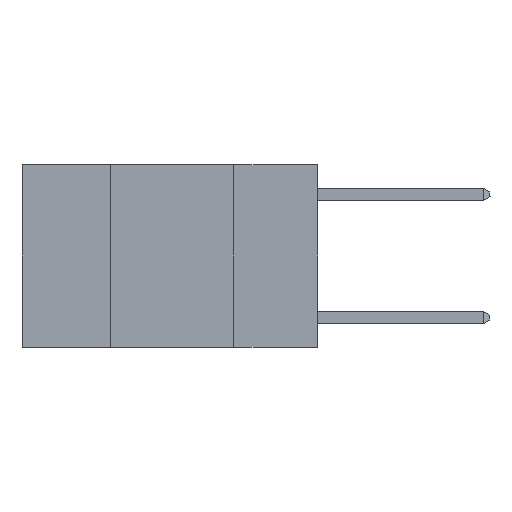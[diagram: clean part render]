
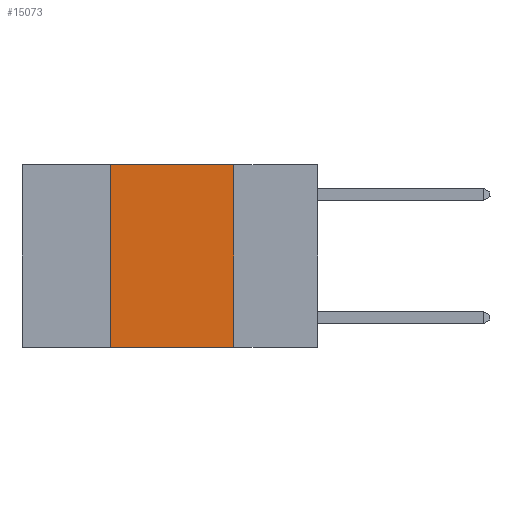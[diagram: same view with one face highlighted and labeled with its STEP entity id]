
A CAD part, left-side view. The second image highlights one B-rep face of the part: STEP entity #15073.
In plain terms, the highlighted planar face has unit normal (-1, 0, 0).
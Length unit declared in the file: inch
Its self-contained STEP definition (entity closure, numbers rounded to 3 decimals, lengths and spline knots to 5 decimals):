
#300 = VECTOR ( 'NONE', #2302, 39.37008 ) ;
#547 = EDGE_CURVE ( 'NONE', #1312, #9649, #878, .T. ) ;
#878 = LINE ( 'NONE', #14777, #6527 ) ;
#1312 = VERTEX_POINT ( 'NONE', #2654 ) ;
#1399 = EDGE_CURVE ( 'NONE', #7088, #1312, #10893, .T. ) ;
#1796 = CARTESIAN_POINT ( 'NONE',  ( 0., 0.6, -0.37 ) ) ;
#2073 = ORIENTED_EDGE ( 'NONE', *, *, #9136, .T. ) ;
#2124 = ORIENTED_EDGE ( 'NONE', *, *, #1399, .F. ) ;
#2302 = DIRECTION ( 'NONE',  ( 0., -1., 0. ) ) ;
#2654 = CARTESIAN_POINT ( 'NONE',  ( 0., 0.17, 0. ) ) ;
#2796 = EDGE_CURVE ( 'NONE', #14034, #7088, #12800, .T. ) ;
#3447 = DIRECTION ( 'NONE',  ( 0., 0., 1. ) ) ;
#3804 = AXIS2_PLACEMENT_3D ( 'NONE', #9010, #4332, #12640 ) ;
#4332 = DIRECTION ( 'NONE',  ( 1., 0., 0. ) ) ;
#4443 = EDGE_LOOP ( 'NONE', ( #9001, #2124, #13896, #2073 ) ) ;
#5183 = DIRECTION ( 'NONE',  ( 0., 0., -1. ) ) ;
#6338 = CARTESIAN_POINT ( 'NONE',  ( 0., 0.42, 0. ) ) ;
#6527 = VECTOR ( 'NONE', #5183, 39.37008 ) ;
#7088 = VERTEX_POINT ( 'NONE', #8324 ) ;
#7372 = VECTOR ( 'NONE', #12510, 39.37008 ) ;
#7829 = PLANE ( 'NONE',  #3804 ) ;
#8324 = CARTESIAN_POINT ( 'NONE',  ( 0., 0.42, 0. ) ) ;
#9001 = ORIENTED_EDGE ( 'NONE', *, *, #547, .F. ) ;
#9010 = CARTESIAN_POINT ( 'NONE',  ( 0., 0.6, 0. ) ) ;
#9136 = EDGE_CURVE ( 'NONE', #14034, #9649, #10462, .T. ) ;
#9571 = VECTOR ( 'NONE', #3447, 39.37008 ) ;
#9649 = VERTEX_POINT ( 'NONE', #13861 ) ;
#10275 = FACE_OUTER_BOUND ( 'NONE', #4443, .T. ) ;
#10462 = LINE ( 'NONE', #1796, #7372 ) ;
#10893 = LINE ( 'NONE', #11881, #300 ) ;
#11881 = CARTESIAN_POINT ( 'NONE',  ( 0., 0.6, 0. ) ) ;
#12510 = DIRECTION ( 'NONE',  ( 0., -1., 0. ) ) ;
#12640 = DIRECTION ( 'NONE',  ( 0., 0., -1. ) ) ;
#12800 = LINE ( 'NONE', #6338, #9571 ) ;
#13861 = CARTESIAN_POINT ( 'NONE',  ( 0., 0.17, -0.37 ) ) ;
#13896 = ORIENTED_EDGE ( 'NONE', *, *, #2796, .F. ) ;
#14034 = VERTEX_POINT ( 'NONE', #14893 ) ;
#14777 = CARTESIAN_POINT ( 'NONE',  ( 0., 0.17, 0. ) ) ;
#14893 = CARTESIAN_POINT ( 'NONE',  ( 0., 0.42, -0.37 ) ) ;
#15073 = ADVANCED_FACE ( 'NONE', ( #10275 ), #7829, .F. ) ;
